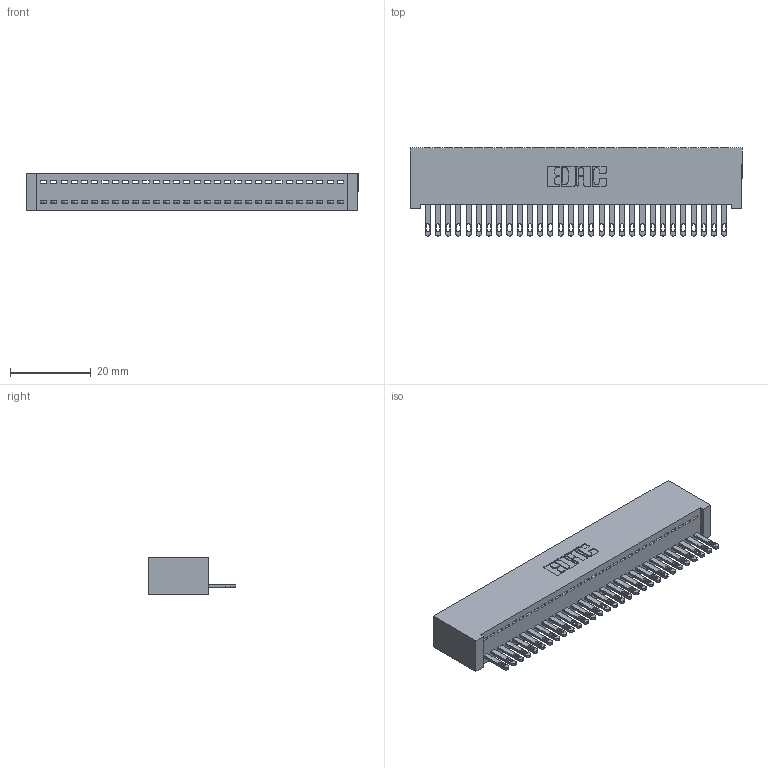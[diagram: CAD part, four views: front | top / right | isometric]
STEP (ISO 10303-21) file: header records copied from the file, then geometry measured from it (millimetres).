
FILE_DESCRIPTION (( 'STEP AP203' ), '1' );
FILE_NAME ('342-030-500-101.STEP', '2019-10-02T04:04:22', ( '' ), ( '' ), 'SwSTEP 2.0', 'SolidWorks 2016', '' );
FILE_SCHEMA (( 'CONFIG_CONTROL_DESIGN' ));
Length unit declared in the file: inch
Products named in the file (3): 342 Part_Lugless; 345-292-001_345-293-100; 342-030-500-101
Assembly tree (31 placements, depth 2):
  342-030-500-101
    342 Part_Lugless
    345-292-001_345-293-100  x30
Bounding box: 82.45 x 21.85 x 9.4 mm (x, y, z)
Volume: 7612.4 mm3; surface area: 11336.8 mm2
Topology: 31 solids, 31 shells, 1722 faces, 5315 edges, 3542 vertices
Faces by surface type: plane 1142, cylinder 580
Entity records: 19413 total; most frequent: CARTESIAN_POINT 3356, ORIENTED_EDGE 3322, DIRECTION 2849, EDGE_CURVE 1661, LINE 1537, VECTOR 1537, VERTEX_POINT 1106, AXIS2_PLACEMENT_3D 656
